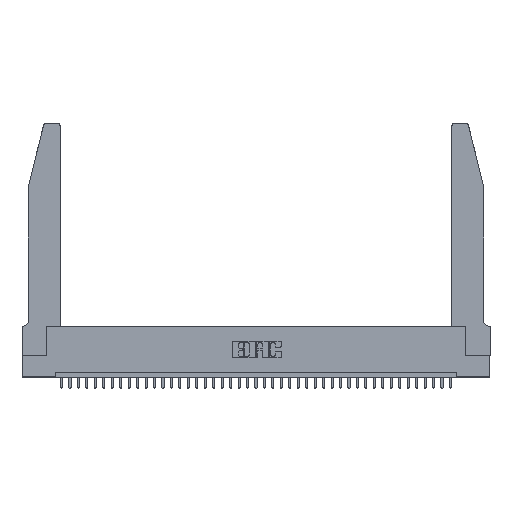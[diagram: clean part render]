
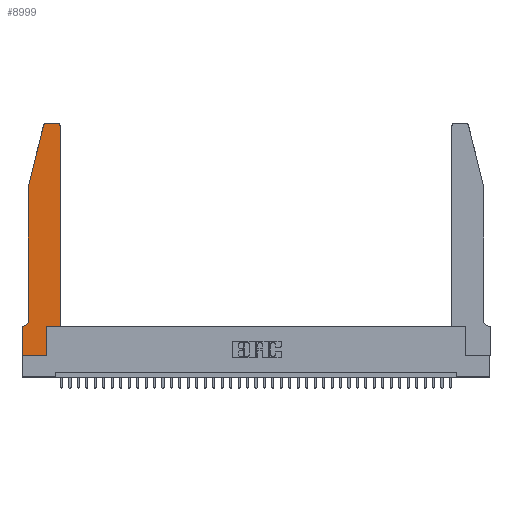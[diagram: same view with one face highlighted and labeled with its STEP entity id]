
A CAD part, top view. The second image highlights one B-rep face of the part: STEP entity #8999.
In plain terms, the highlighted planar face has unit normal (0, 0, 1).
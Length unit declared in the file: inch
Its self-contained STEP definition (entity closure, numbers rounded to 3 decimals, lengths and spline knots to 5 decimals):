
#76 = CIRCLE ( 'NONE', #17536, 0.07 ) ;
#354 = CIRCLE ( 'NONE', #7843, 0.03 ) ;
#864 = DIRECTION ( 'NONE',  ( 0., -1., 0. ) ) ;
#1175 = DIRECTION ( 'NONE',  ( 1., 0., 0. ) ) ;
#1620 = CARTESIAN_POINT ( 'NONE',  ( 0., 0., 0.37 ) ) ;
#2047 = CARTESIAN_POINT ( 'NONE',  ( 0.2865, 0.35, 0.37 ) ) ;
#2304 = DIRECTION ( 'NONE',  ( 0., 1., 0. ) ) ;
#2442 = VERTEX_POINT ( 'NONE', #2047 ) ;
#3024 = DIRECTION ( 'NONE',  ( 1., 0., 0. ) ) ;
#3282 = CARTESIAN_POINT ( 'NONE',  ( 0.0055, 0.42, 0.37 ) ) ;
#3645 = EDGE_CURVE ( 'NONE', #37594, #9245, #19493, .T. ) ;
#5179 = VERTEX_POINT ( 'NONE', #35983 ) ;
#5494 = VECTOR ( 'NONE', #24053, 39.37008 ) ;
#6106 = EDGE_CURVE ( 'NONE', #9245, #8229, #76, .T. ) ;
#6117 = ORIENTED_EDGE ( 'NONE', *, *, #18680, .T. ) ;
#6177 = DIRECTION ( 'NONE',  ( 0., 0., 1. ) ) ;
#6606 = VECTOR ( 'NONE', #864, 39.37008 ) ;
#6687 = DIRECTION ( 'NONE',  ( -1., 0., 0. ) ) ;
#6858 = CARTESIAN_POINT ( 'NONE',  ( 0.0755, 2., 0.37 ) ) ;
#7502 = DIRECTION ( 'NONE',  ( 0., -1., 0. ) ) ;
#7795 = DIRECTION ( 'NONE',  ( -0.239, -0.971, 0. ) ) ;
#7843 = AXIS2_PLACEMENT_3D ( 'NONE', #9077, #6177, #24416 ) ;
#8229 = VERTEX_POINT ( 'NONE', #21457 ) ;
#8811 = VECTOR ( 'NONE', #6687, 39.37008 ) ;
#8999 = ADVANCED_FACE ( 'NONE', ( #22741 ), #21537, .T. ) ;
#9077 = CARTESIAN_POINT ( 'NONE',  ( 0.284, 2.72, 0.37 ) ) ;
#9245 = VERTEX_POINT ( 'NONE', #32044 ) ;
#9863 = EDGE_CURVE ( 'NONE', #30811, #27043, #29825, .T. ) ;
#9901 = DIRECTION ( 'NONE',  ( 0., 0., -1. ) ) ;
#9986 = VECTOR ( 'NONE', #2304, 39.37008 ) ;
#10322 = EDGE_CURVE ( 'NONE', #34001, #37594, #24551, .T. ) ;
#10482 = LINE ( 'NONE', #34849, #9986 ) ;
#12290 = AXIS2_PLACEMENT_3D ( 'NONE', #25818, #35027, #1175 ) ;
#12941 = LINE ( 'NONE', #35882, #20580 ) ;
#13092 = VECTOR ( 'NONE', #7795, 39.37008 ) ;
#16322 = AXIS2_PLACEMENT_3D ( 'NONE', #27565, #33420, #3024 ) ;
#16484 = LINE ( 'NONE', #22896, #32266 ) ;
#17147 = EDGE_CURVE ( 'NONE', #24919, #30811, #34201, .T. ) ;
#17536 = AXIS2_PLACEMENT_3D ( 'NONE', #3282, #9901, #24840 ) ;
#17847 = LINE ( 'NONE', #28703, #26938 ) ;
#18076 = EDGE_CURVE ( 'NONE', #26543, #24919, #10482, .T. ) ;
#18680 = EDGE_CURVE ( 'NONE', #2442, #26543, #39048, .T. ) ;
#19493 = LINE ( 'NONE', #6858, #6606 ) ;
#19688 = CARTESIAN_POINT ( 'NONE',  ( 0.4505, 0.35, 0.37 ) ) ;
#20578 = CARTESIAN_POINT ( 'NONE',  ( 0., 0.35, 0.37 ) ) ;
#20580 = VECTOR ( 'NONE', #23470, 39.37008 ) ;
#20915 = ORIENTED_EDGE ( 'NONE', *, *, #23305, .T. ) ;
#20982 = ORIENTED_EDGE ( 'NONE', *, *, #38317, .T. ) ;
#21457 = CARTESIAN_POINT ( 'NONE',  ( 0.0055, 0.35, 0.37 ) ) ;
#21518 = CARTESIAN_POINT ( 'NONE',  ( 0.284, 2.75, 0.37 ) ) ;
#21537 = PLANE ( 'NONE',  #16322 ) ;
#21637 = VERTEX_POINT ( 'NONE', #20578 ) ;
#22380 = VECTOR ( 'NONE', #29347, 39.37008 ) ;
#22741 = FACE_OUTER_BOUND ( 'NONE', #30328, .T. ) ;
#22896 = CARTESIAN_POINT ( 'NONE',  ( 0.2865, 0.35, 0.37 ) ) ;
#23305 = EDGE_CURVE ( 'NONE', #5179, #2442, #16484, .T. ) ;
#23470 = DIRECTION ( 'NONE',  ( -1., 0., 0. ) ) ;
#23555 = ORIENTED_EDGE ( 'NONE', *, *, #30552, .T. ) ;
#24053 = DIRECTION ( 'NONE',  ( 1., 0., 0. ) ) ;
#24416 = DIRECTION ( 'NONE',  ( 1., 0., 0. ) ) ;
#24551 = LINE ( 'NONE', #29136, #13092 ) ;
#24840 = DIRECTION ( 'NONE',  ( -1., 0., 0. ) ) ;
#24919 = VERTEX_POINT ( 'NONE', #34636 ) ;
#25664 = CARTESIAN_POINT ( 'NONE',  ( 0.4205, 2.75, 0.37 ) ) ;
#25784 = EDGE_CURVE ( 'NONE', #27043, #34001, #354, .T. ) ;
#25818 = CARTESIAN_POINT ( 'NONE',  ( 0.4205, 2.72, 0.37 ) ) ;
#26239 = DIRECTION ( 'NONE',  ( 0., 1., 0. ) ) ;
#26543 = VERTEX_POINT ( 'NONE', #19688 ) ;
#26938 = VECTOR ( 'NONE', #7502, 39.37008 ) ;
#27043 = VERTEX_POINT ( 'NONE', #21518 ) ;
#27565 = CARTESIAN_POINT ( 'NONE',  ( 0., 0.35, 0.37 ) ) ;
#28172 = ORIENTED_EDGE ( 'NONE', *, *, #10322, .T. ) ;
#28309 = ORIENTED_EDGE ( 'NONE', *, *, #17147, .T. ) ;
#28703 = CARTESIAN_POINT ( 'NONE',  ( 0., 0., 0.37 ) ) ;
#29087 = CARTESIAN_POINT ( 'NONE',  ( 0.4505, 0.35, 0.37 ) ) ;
#29136 = CARTESIAN_POINT ( 'NONE',  ( 0.0755, 2., 0.37 ) ) ;
#29151 = VERTEX_POINT ( 'NONE', #29339 ) ;
#29189 = ORIENTED_EDGE ( 'NONE', *, *, #9863, .T. ) ;
#29339 = CARTESIAN_POINT ( 'NONE',  ( 0., 0., 0.37 ) ) ;
#29347 = DIRECTION ( 'NONE',  ( 1., 0., 0. ) ) ;
#29825 = LINE ( 'NONE', #31201, #8811 ) ;
#30328 = EDGE_LOOP ( 'NONE', ( #29189, #39251, #28172, #31796, #33205, #20982, #33647, #23555, #20915, #6117, #35121, #28309 ) ) ;
#30482 = EDGE_CURVE ( 'NONE', #21637, #29151, #17847, .T. ) ;
#30552 = EDGE_CURVE ( 'NONE', #29151, #5179, #30760, .T. ) ;
#30760 = LINE ( 'NONE', #1620, #5494 ) ;
#30811 = VERTEX_POINT ( 'NONE', #25664 ) ;
#31201 = CARTESIAN_POINT ( 'NONE',  ( 0.2605, 2.75, 0.37 ) ) ;
#31796 = ORIENTED_EDGE ( 'NONE', *, *, #3645, .T. ) ;
#32044 = CARTESIAN_POINT ( 'NONE',  ( 0.0755, 0.42, 0.37 ) ) ;
#32266 = VECTOR ( 'NONE', #26239, 39.37008 ) ;
#33205 = ORIENTED_EDGE ( 'NONE', *, *, #6106, .T. ) ;
#33420 = DIRECTION ( 'NONE',  ( 0., 0., 1. ) ) ;
#33647 = ORIENTED_EDGE ( 'NONE', *, *, #30482, .T. ) ;
#34001 = VERTEX_POINT ( 'NONE', #39344 ) ;
#34201 = CIRCLE ( 'NONE', #12290, 0.03 ) ;
#34636 = CARTESIAN_POINT ( 'NONE',  ( 0.4505, 2.72, 0.37 ) ) ;
#34849 = CARTESIAN_POINT ( 'NONE',  ( 0.4505, 0.35, 0.37 ) ) ;
#34878 = CARTESIAN_POINT ( 'NONE',  ( 0.0755, 2., 0.37 ) ) ;
#35027 = DIRECTION ( 'NONE',  ( 0., 0., 1. ) ) ;
#35121 = ORIENTED_EDGE ( 'NONE', *, *, #18076, .T. ) ;
#35882 = CARTESIAN_POINT ( 'NONE',  ( 0.0755, 0.35, 0.37 ) ) ;
#35983 = CARTESIAN_POINT ( 'NONE',  ( 0.2865, 0., 0.37 ) ) ;
#37594 = VERTEX_POINT ( 'NONE', #34878 ) ;
#38317 = EDGE_CURVE ( 'NONE', #8229, #21637, #12941, .T. ) ;
#39048 = LINE ( 'NONE', #29087, #22380 ) ;
#39251 = ORIENTED_EDGE ( 'NONE', *, *, #25784, .T. ) ;
#39344 = CARTESIAN_POINT ( 'NONE',  ( 0.25487, 2.72718, 0.37 ) ) ;
